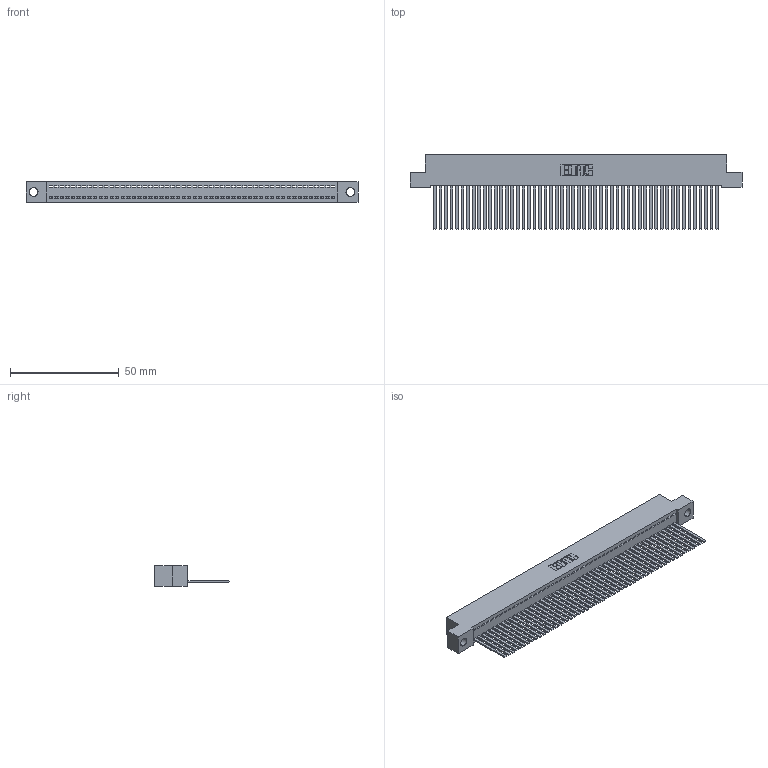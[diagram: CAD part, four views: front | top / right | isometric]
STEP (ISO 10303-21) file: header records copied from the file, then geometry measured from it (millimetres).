
FILE_DESCRIPTION (( 'STEP AP203' ), '1' );
FILE_NAME ('392-052-544-104.STEP', '2018-08-17T05:53:49', ( '' ), ( '' ), 'SwSTEP 2.0', 'SolidWorks 2016', '' );
FILE_SCHEMA (( 'CONFIG_CONTROL_DESIGN' ));
Length unit declared in the file: inch
Products named in the file (3): 342 Part_.156 TH; 345-292-001_345-293-144; 392-052-544-104
Assembly tree (53 placements, depth 2):
  392-052-544-104
    342 Part_.156 TH
    345-292-001_345-293-144  x52
Bounding box: 152.4 x 34.3 x 9.4 mm (x, y, z)
Volume: 13914.5 mm3; surface area: 22152.3 mm2
Topology: 53 solids, 53 shells, 2814 faces, 8515 edges, 5606 vertices
Faces by surface type: plane 2042, cylinder 772
Entity records: 30183 total; most frequent: CARTESIAN_POINT 5210, ORIENTED_EDGE 5198, DIRECTION 4371, EDGE_CURVE 2599, LINE 2475, VECTOR 2475, VERTEX_POINT 1730, AXIS2_PLACEMENT_3D 948
